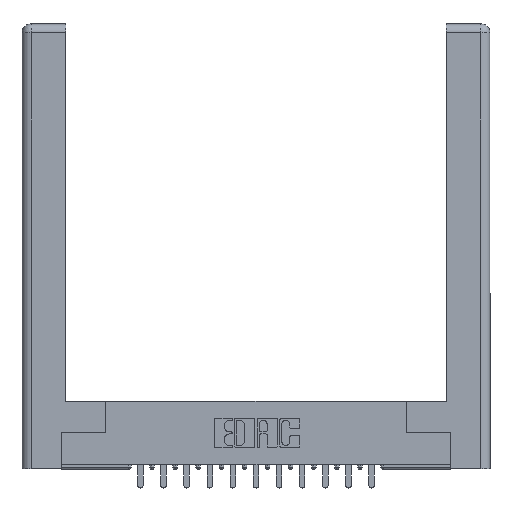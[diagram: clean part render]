
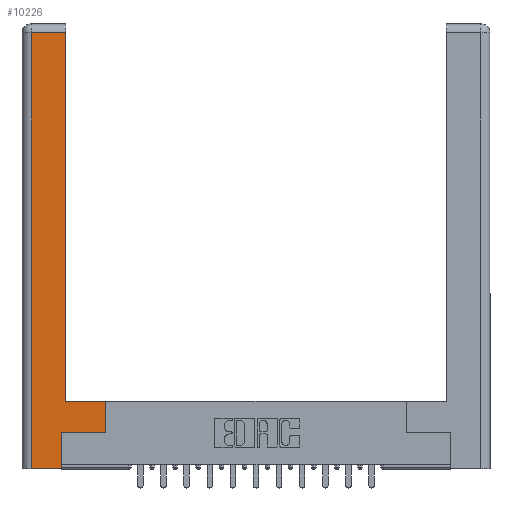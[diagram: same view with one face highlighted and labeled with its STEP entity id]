
A CAD part, top view. The second image highlights one B-rep face of the part: STEP entity #10226.
In plain terms, the highlighted planar face has unit normal (0, 0, 1).
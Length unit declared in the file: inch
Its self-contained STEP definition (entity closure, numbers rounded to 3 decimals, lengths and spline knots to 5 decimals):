
#55 = CARTESIAN_POINT ( 'NONE',  ( 0.565, 0.245, 0. ) ) ;
#1100 = VERTEX_POINT ( 'NONE', #11509 ) ;
#1448 = ORIENTED_EDGE ( 'NONE', *, *, #14641, .T. ) ;
#1450 = AXIS2_PLACEMENT_3D ( 'NONE', #16126, #14905, #4556 ) ;
#1538 = FACE_OUTER_BOUND ( 'NONE', #4780, .T. ) ;
#1777 = EDGE_CURVE ( 'NONE', #10147, #3275, #10017, .T. ) ;
#2255 = ORIENTED_EDGE ( 'NONE', *, *, #14525, .T. ) ;
#2303 = CARTESIAN_POINT ( 'NONE',  ( 0.0615, 0., 0. ) ) ;
#2701 = DIRECTION ( 'NONE',  ( 1., 0., 0. ) ) ;
#2838 = CARTESIAN_POINT ( 'NONE',  ( 0.265, 0.245, 0. ) ) ;
#2991 = DIRECTION ( 'NONE',  ( 0., 1., 0. ) ) ;
#3275 = VERTEX_POINT ( 'NONE', #8768 ) ;
#3677 = CARTESIAN_POINT ( 'NONE',  ( 0.295, 3., 0. ) ) ;
#4225 = VECTOR ( 'NONE', #11649, 39.37008 ) ;
#4467 = EDGE_CURVE ( 'NONE', #3275, #1100, #10329, .T. ) ;
#4515 = CARTESIAN_POINT ( 'NONE',  ( 0.295, 0.45, 0. ) ) ;
#4555 = DIRECTION ( 'NONE',  ( 0., -1., 0. ) ) ;
#4556 = DIRECTION ( 'NONE',  ( -1., 0., 0. ) ) ;
#4780 = EDGE_LOOP ( 'NONE', ( #2255, #10273, #13498, #9783, #5486, #8302, #9704, #1448 ) ) ;
#4971 = VERTEX_POINT ( 'NONE', #12077 ) ;
#5188 = VERTEX_POINT ( 'NONE', #8233 ) ;
#5212 = LINE ( 'NONE', #16301, #7453 ) ;
#5486 = ORIENTED_EDGE ( 'NONE', *, *, #1777, .T. ) ;
#6513 = EDGE_CURVE ( 'NONE', #5188, #14644, #16106, .T. ) ;
#6706 = VERTEX_POINT ( 'NONE', #10993 ) ;
#6952 = CARTESIAN_POINT ( 'NONE',  ( 0.565, 0.45, 0. ) ) ;
#6996 = VECTOR ( 'NONE', #11242, 39.37008 ) ;
#7123 = EDGE_CURVE ( 'NONE', #1100, #6706, #10610, .T. ) ;
#7374 = VECTOR ( 'NONE', #12365, 39.37008 ) ;
#7453 = VECTOR ( 'NONE', #4555, 39.37008 ) ;
#8078 = VECTOR ( 'NONE', #2701, 39.37008 ) ;
#8233 = CARTESIAN_POINT ( 'NONE',  ( 0.295, 2.94, 0. ) ) ;
#8302 = ORIENTED_EDGE ( 'NONE', *, *, #4467, .T. ) ;
#8397 = PLANE ( 'NONE',  #1450 ) ;
#8466 = LINE ( 'NONE', #3677, #8889 ) ;
#8661 = CARTESIAN_POINT ( 'NONE',  ( 0.0615, 2.94, 0. ) ) ;
#8768 = CARTESIAN_POINT ( 'NONE',  ( 0.265, 0.245, 0. ) ) ;
#8889 = VECTOR ( 'NONE', #10118, 39.37008 ) ;
#9475 = LINE ( 'NONE', #4515, #10279 ) ;
#9704 = ORIENTED_EDGE ( 'NONE', *, *, #7123, .T. ) ;
#9783 = ORIENTED_EDGE ( 'NONE', *, *, #10606, .T. ) ;
#10017 = LINE ( 'NONE', #2838, #7374 ) ;
#10118 = DIRECTION ( 'NONE',  ( 0., 1., 0. ) ) ;
#10147 = VERTEX_POINT ( 'NONE', #15814 ) ;
#10226 = ADVANCED_FACE ( 'NONE', ( #1538 ), #8397, .F. ) ;
#10273 = ORIENTED_EDGE ( 'NONE', *, *, #6513, .T. ) ;
#10279 = VECTOR ( 'NONE', #16608, 39.37008 ) ;
#10329 = LINE ( 'NONE', #55, #4225 ) ;
#10606 = EDGE_CURVE ( 'NONE', #13292, #10147, #14965, .T. ) ;
#10610 = LINE ( 'NONE', #6952, #16292 ) ;
#10993 = CARTESIAN_POINT ( 'NONE',  ( 0.565, 0.45, 0. ) ) ;
#11242 = DIRECTION ( 'NONE',  ( -1., 0., 0. ) ) ;
#11455 = EDGE_CURVE ( 'NONE', #14644, #13292, #5212, .T. ) ;
#11509 = CARTESIAN_POINT ( 'NONE',  ( 0.565, 0.245, 0. ) ) ;
#11649 = DIRECTION ( 'NONE',  ( 1., 0., 0. ) ) ;
#11723 = CARTESIAN_POINT ( 'NONE',  ( 0.265, 0., 0. ) ) ;
#12077 = CARTESIAN_POINT ( 'NONE',  ( 0.295, 0.45, 0. ) ) ;
#12365 = DIRECTION ( 'NONE',  ( 0., 1., 0. ) ) ;
#13292 = VERTEX_POINT ( 'NONE', #2303 ) ;
#13498 = ORIENTED_EDGE ( 'NONE', *, *, #11455, .T. ) ;
#13952 = CARTESIAN_POINT ( 'NONE',  ( 0.0615, 2.94, 0. ) ) ;
#14525 = EDGE_CURVE ( 'NONE', #4971, #5188, #8466, .T. ) ;
#14641 = EDGE_CURVE ( 'NONE', #6706, #4971, #9475, .T. ) ;
#14644 = VERTEX_POINT ( 'NONE', #13952 ) ;
#14905 = DIRECTION ( 'NONE',  ( 0., 0., -1. ) ) ;
#14965 = LINE ( 'NONE', #11723, #8078 ) ;
#15814 = CARTESIAN_POINT ( 'NONE',  ( 0.265, 0., 0. ) ) ;
#16106 = LINE ( 'NONE', #8661, #6996 ) ;
#16126 = CARTESIAN_POINT ( 'NONE',  ( 0., 0., 0. ) ) ;
#16292 = VECTOR ( 'NONE', #2991, 39.37008 ) ;
#16301 = CARTESIAN_POINT ( 'NONE',  ( 0.0615, 0., 0. ) ) ;
#16608 = DIRECTION ( 'NONE',  ( -1., 0., 0. ) ) ;
